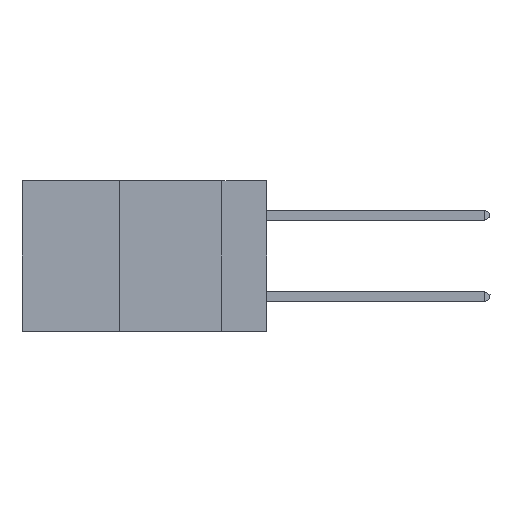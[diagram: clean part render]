
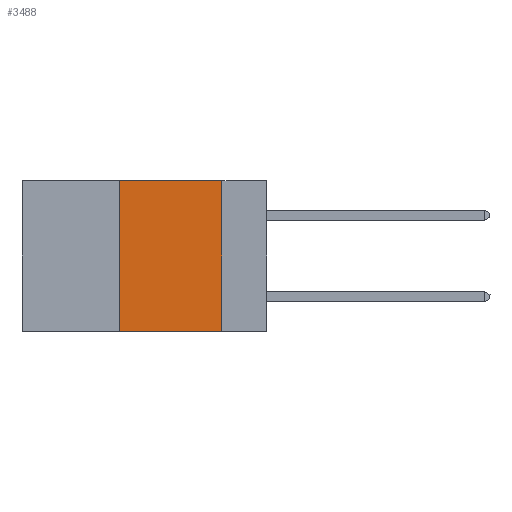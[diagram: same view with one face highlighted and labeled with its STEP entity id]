
A CAD part, left-side view. The second image highlights one B-rep face of the part: STEP entity #3488.
In plain terms, the highlighted planar face has unit normal (-1, 0, 0).
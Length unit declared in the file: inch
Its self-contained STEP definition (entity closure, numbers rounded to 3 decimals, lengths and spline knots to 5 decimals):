
#95 = LINE ( 'NONE', #4087, #7039 ) ;
#187 = DIRECTION ( 'NONE',  ( 0., -1., 0. ) ) ;
#274 = DIRECTION ( 'NONE',  ( 0., 0., 1. ) ) ;
#360 = VERTEX_POINT ( 'NONE', #9621 ) ;
#730 = DIRECTION ( 'NONE',  ( 0., 0., -1. ) ) ;
#733 = DIRECTION ( 'NONE',  ( 0., 0., -1. ) ) ;
#751 = LINE ( 'NONE', #2918, #5619 ) ;
#789 = VECTOR ( 'NONE', #730, 39.37008 ) ;
#2401 = EDGE_CURVE ( 'NONE', #7148, #360, #7736, .T. ) ;
#2918 = CARTESIAN_POINT ( 'NONE',  ( 0., 0.6, -0.37 ) ) ;
#3115 = DIRECTION ( 'NONE',  ( 0., -1., 0. ) ) ;
#3149 = CARTESIAN_POINT ( 'NONE',  ( 0., 0.11, 0. ) ) ;
#3288 = EDGE_CURVE ( 'NONE', #5978, #6963, #8258, .T. ) ;
#3488 = ADVANCED_FACE ( 'NONE', ( #6929 ), #10076, .F. ) ;
#4087 = CARTESIAN_POINT ( 'NONE',  ( 0., 0.6, 0. ) ) ;
#4475 = ORIENTED_EDGE ( 'NONE', *, *, #5790, .F. ) ;
#4746 = AXIS2_PLACEMENT_3D ( 'NONE', #6777, #5958, #733 ) ;
#5041 = ORIENTED_EDGE ( 'NONE', *, *, #2401, .F. ) ;
#5619 = VECTOR ( 'NONE', #3115, 39.37008 ) ;
#5790 = EDGE_CURVE ( 'NONE', #6963, #7148, #95, .T. ) ;
#5909 = ORIENTED_EDGE ( 'NONE', *, *, #8593, .T. ) ;
#5958 = DIRECTION ( 'NONE',  ( 1., 0., 0. ) ) ;
#5978 = VERTEX_POINT ( 'NONE', #9824 ) ;
#6343 = CARTESIAN_POINT ( 'NONE',  ( 0., 0.11, 0. ) ) ;
#6777 = CARTESIAN_POINT ( 'NONE',  ( 0., 0.6, 0. ) ) ;
#6856 = ORIENTED_EDGE ( 'NONE', *, *, #3288, .F. ) ;
#6902 = VECTOR ( 'NONE', #274, 39.37008 ) ;
#6929 = FACE_OUTER_BOUND ( 'NONE', #9023, .T. ) ;
#6963 = VERTEX_POINT ( 'NONE', #8393 ) ;
#7039 = VECTOR ( 'NONE', #187, 39.37008 ) ;
#7148 = VERTEX_POINT ( 'NONE', #6343 ) ;
#7385 = CARTESIAN_POINT ( 'NONE',  ( 0., 0.36, 0. ) ) ;
#7736 = LINE ( 'NONE', #3149, #789 ) ;
#8258 = LINE ( 'NONE', #7385, #6902 ) ;
#8393 = CARTESIAN_POINT ( 'NONE',  ( 0., 0.36, 0. ) ) ;
#8593 = EDGE_CURVE ( 'NONE', #5978, #360, #751, .T. ) ;
#9023 = EDGE_LOOP ( 'NONE', ( #5041, #4475, #6856, #5909 ) ) ;
#9621 = CARTESIAN_POINT ( 'NONE',  ( 0., 0.11, -0.37 ) ) ;
#9824 = CARTESIAN_POINT ( 'NONE',  ( 0., 0.36, -0.37 ) ) ;
#10076 = PLANE ( 'NONE',  #4746 ) ;
